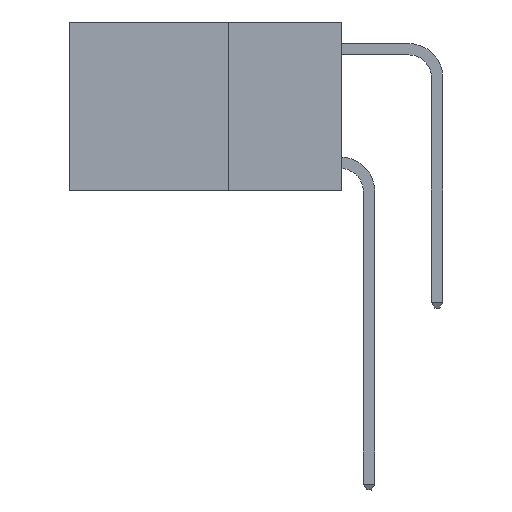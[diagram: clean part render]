
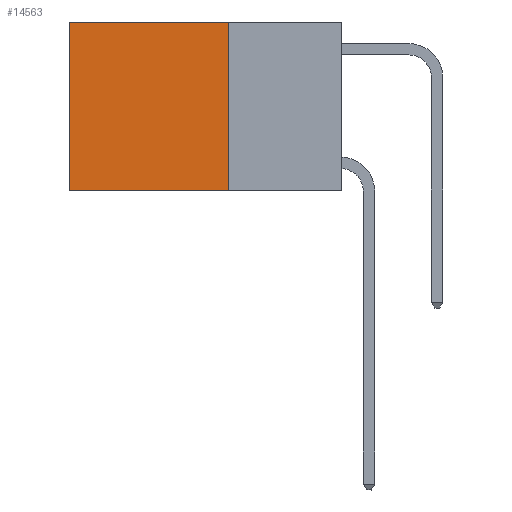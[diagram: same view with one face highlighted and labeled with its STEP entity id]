
A CAD part, left-side view. The second image highlights one B-rep face of the part: STEP entity #14563.
In plain terms, the highlighted planar face has unit normal (-1, 0, 0).
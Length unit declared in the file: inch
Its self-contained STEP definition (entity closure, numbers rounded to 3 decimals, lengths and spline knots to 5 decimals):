
#1236 = DIRECTION ( 'NONE',  ( 0., 0., -1. ) ) ;
#1378 = VECTOR ( 'NONE', #1236, 39.37008 ) ;
#1588 = CARTESIAN_POINT ( 'NONE',  ( 0.2625, 0.6, -0.37 ) ) ;
#1815 = ORIENTED_EDGE ( 'NONE', *, *, #5935, .F. ) ;
#2132 = CARTESIAN_POINT ( 'NONE',  ( 0.2625, 0.25, 0. ) ) ;
#3052 = VERTEX_POINT ( 'NONE', #12160 ) ;
#3460 = FACE_OUTER_BOUND ( 'NONE', #4355, .T. ) ;
#3733 = VECTOR ( 'NONE', #12599, 39.37008 ) ;
#3909 = VECTOR ( 'NONE', #11279, 39.37008 ) ;
#3972 = VECTOR ( 'NONE', #17363, 39.37008 ) ;
#4178 = VERTEX_POINT ( 'NONE', #10245 ) ;
#4355 = EDGE_LOOP ( 'NONE', ( #8899, #12108, #1815, #9503 ) ) ;
#4440 = LINE ( 'NONE', #11367, #3733 ) ;
#4902 = LINE ( 'NONE', #2132, #3972 ) ;
#5935 = EDGE_CURVE ( 'NONE', #3052, #4178, #13657, .T. ) ;
#6479 = VERTEX_POINT ( 'NONE', #14567 ) ;
#6663 = CARTESIAN_POINT ( 'NONE',  ( 0.2625, 0.25, -0.37 ) ) ;
#6941 = EDGE_CURVE ( 'NONE', #6479, #18288, #4440, .T. ) ;
#7126 = CARTESIAN_POINT ( 'NONE',  ( 0.2625, 0.25, 0. ) ) ;
#8366 = LINE ( 'NONE', #6663, #3909 ) ;
#8899 = ORIENTED_EDGE ( 'NONE', *, *, #6941, .T. ) ;
#9503 = ORIENTED_EDGE ( 'NONE', *, *, #14337, .T. ) ;
#9711 = EDGE_CURVE ( 'NONE', #4178, #18288, #8366, .T. ) ;
#10245 = CARTESIAN_POINT ( 'NONE',  ( 0.2625, 0.25, -0.37 ) ) ;
#10448 = CARTESIAN_POINT ( 'NONE',  ( 0.2625, 0.25, 0. ) ) ;
#11279 = DIRECTION ( 'NONE',  ( 0., 1., 0. ) ) ;
#11367 = CARTESIAN_POINT ( 'NONE',  ( 0.2625, 0.6, 0. ) ) ;
#11955 = DIRECTION ( 'NONE',  ( 1., 0., 0. ) ) ;
#12108 = ORIENTED_EDGE ( 'NONE', *, *, #9711, .F. ) ;
#12160 = CARTESIAN_POINT ( 'NONE',  ( 0.2625, 0.25, 0. ) ) ;
#12599 = DIRECTION ( 'NONE',  ( 0., 0., -1. ) ) ;
#13270 = PLANE ( 'NONE',  #18794 ) ;
#13657 = LINE ( 'NONE', #7126, #1378 ) ;
#14337 = EDGE_CURVE ( 'NONE', #3052, #6479, #4902, .T. ) ;
#14563 = ADVANCED_FACE ( 'NONE', ( #3460 ), #13270, .F. ) ;
#14567 = CARTESIAN_POINT ( 'NONE',  ( 0.2625, 0.6, 0. ) ) ;
#14827 = DIRECTION ( 'NONE',  ( 0., 0., -1. ) ) ;
#17363 = DIRECTION ( 'NONE',  ( 0., 1., 0. ) ) ;
#18288 = VERTEX_POINT ( 'NONE', #1588 ) ;
#18794 = AXIS2_PLACEMENT_3D ( 'NONE', #10448, #11955, #14827 ) ;
